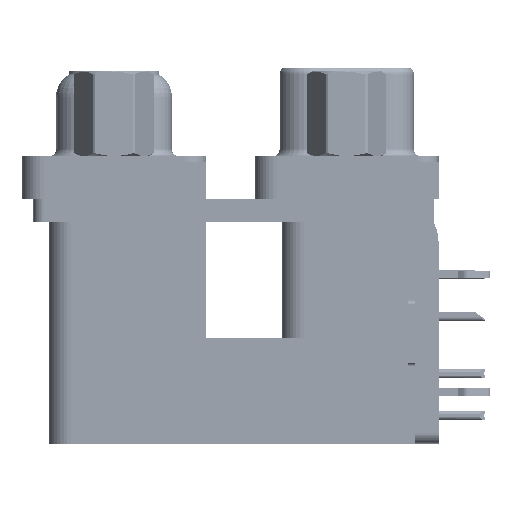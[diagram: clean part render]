
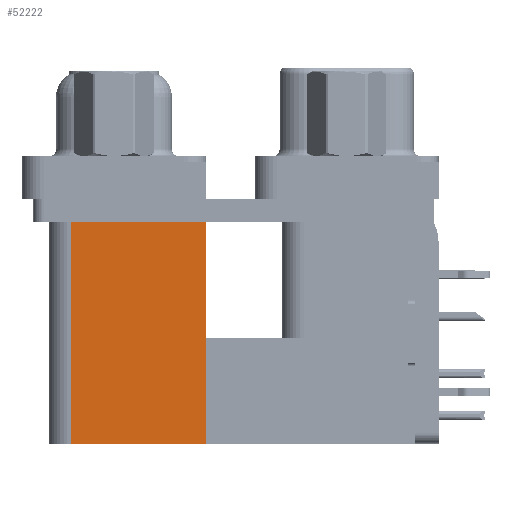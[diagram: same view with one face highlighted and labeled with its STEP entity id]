
A CAD part, left-side view. The second image highlights one B-rep face of the part: STEP entity #52222.
In plain terms, the highlighted planar face has unit normal (-1, 0, 0).
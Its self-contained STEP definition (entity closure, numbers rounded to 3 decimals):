
#1910 = VERTEX_POINT ( 'NONE', #59396 ) ;
#3204 = DIRECTION ( 'NONE',  ( 0., 0., 1. ) ) ;
#4684 = PLANE ( 'NONE',  #74760 ) ;
#5345 = LINE ( 'NONE', #74163, #14360 ) ;
#14360 = VECTOR ( 'NONE', #52072, 1000. ) ;
#15710 = EDGE_CURVE ( 'NONE', #31189, #22535, #5345, .T. ) ;
#19915 = LINE ( 'NONE', #65901, #28041 ) ;
#21066 = DIRECTION ( 'NONE',  ( 0., 1., 0. ) ) ;
#22251 = ORIENTED_EDGE ( 'NONE', *, *, #23110, .F. ) ;
#22535 = VERTEX_POINT ( 'NONE', #71355 ) ;
#23110 = EDGE_CURVE ( 'NONE', #40114, #1910, #62473, .T. ) ;
#24378 = CARTESIAN_POINT ( 'NONE',  ( 3.79, 9.6, -2.5 ) ) ;
#26779 = ORIENTED_EDGE ( 'NONE', *, *, #15710, .T. ) ;
#28041 = VECTOR ( 'NONE', #61328, 1000. ) ;
#28388 = ORIENTED_EDGE ( 'NONE', *, *, #74052, .T. ) ;
#30617 = VECTOR ( 'NONE', #3204, 1000. ) ;
#31189 = VERTEX_POINT ( 'NONE', #59872 ) ;
#32076 = CARTESIAN_POINT ( 'NONE',  ( 3.79, 18.8, -19.2 ) ) ;
#39397 = EDGE_CURVE ( 'NONE', #31189, #40114, #19915, .T. ) ;
#40114 = VERTEX_POINT ( 'NONE', #49593 ) ;
#41998 = ORIENTED_EDGE ( 'NONE', *, *, #39397, .F. ) ;
#43802 = VECTOR ( 'NONE', #65035, 1000. ) ;
#45685 = FACE_OUTER_BOUND ( 'NONE', #54273, .T. ) ;
#47137 = LINE ( 'NONE', #24378, #43802 ) ;
#49593 = CARTESIAN_POINT ( 'NONE',  ( 3.79, 18.8, -19.2 ) ) ;
#52072 = DIRECTION ( 'NONE',  ( 0., 0., 1. ) ) ;
#52222 = ADVANCED_FACE ( 'NONE', ( #45685 ), #4684, .F. ) ;
#54273 = EDGE_LOOP ( 'NONE', ( #28388, #22251, #41998, #26779 ) ) ;
#56746 = CARTESIAN_POINT ( 'NONE',  ( 3.79, 9.6, -19.2 ) ) ;
#59396 = CARTESIAN_POINT ( 'NONE',  ( 3.79, 18.8, -2.5 ) ) ;
#59872 = CARTESIAN_POINT ( 'NONE',  ( 3.79, 9.6, -19.2 ) ) ;
#61328 = DIRECTION ( 'NONE',  ( 0., 1., 0. ) ) ;
#62473 = LINE ( 'NONE', #32076, #30617 ) ;
#65035 = DIRECTION ( 'NONE',  ( 0., 1., 0. ) ) ;
#65901 = CARTESIAN_POINT ( 'NONE',  ( 3.79, 9.6, -19.2 ) ) ;
#68921 = DIRECTION ( 'NONE',  ( 1., 0., 0. ) ) ;
#71355 = CARTESIAN_POINT ( 'NONE',  ( 3.79, 9.6, -2.5 ) ) ;
#74052 = EDGE_CURVE ( 'NONE', #22535, #1910, #47137, .T. ) ;
#74163 = CARTESIAN_POINT ( 'NONE',  ( 3.79, 9.6, -19.2 ) ) ;
#74760 = AXIS2_PLACEMENT_3D ( 'NONE', #56746, #68921, #21066 ) ;
